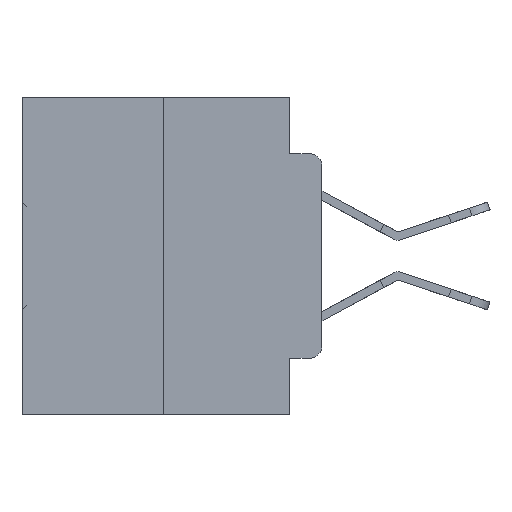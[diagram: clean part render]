
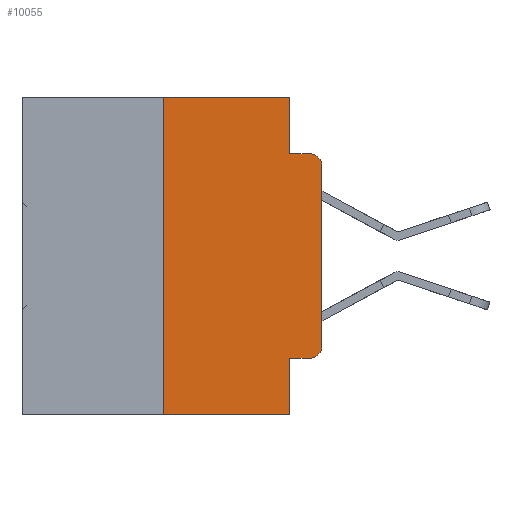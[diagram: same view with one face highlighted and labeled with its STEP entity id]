
A CAD part, left-side view. The second image highlights one B-rep face of the part: STEP entity #10055.
In plain terms, the highlighted planar face has unit normal (-1, 0, 0).
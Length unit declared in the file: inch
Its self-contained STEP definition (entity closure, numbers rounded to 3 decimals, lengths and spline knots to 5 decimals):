
#95 = VECTOR ( 'NONE', #13742, 39.37008 ) ;
#285 = LINE ( 'NONE', #8115, #6824 ) ;
#997 = DIRECTION ( 'NONE',  ( 0., 0., -1. ) ) ;
#1004 = AXIS2_PLACEMENT_3D ( 'NONE', #31628, #31731, #15728 ) ;
#1594 = LINE ( 'NONE', #14963, #7240 ) ;
#1630 = CARTESIAN_POINT ( 'NONE',  ( 0., 0.051, 0. ) ) ;
#1645 = VECTOR ( 'NONE', #19854, 39.37008 ) ;
#3509 = DIRECTION ( 'NONE',  ( 0., -1., 0. ) ) ;
#4352 = EDGE_CURVE ( 'NONE', #29738, #25983, #16354, .T. ) ;
#5220 = DIRECTION ( 'NONE',  ( 0., 0., -1. ) ) ;
#5519 = DIRECTION ( 'NONE',  ( -1., 0., 0. ) ) ;
#6055 = CARTESIAN_POINT ( 'NONE',  ( 0., 0., 0. ) ) ;
#6824 = VECTOR ( 'NONE', #5220, 39.37008 ) ;
#6904 = EDGE_CURVE ( 'NONE', #14923, #12381, #17433, .T. ) ;
#7240 = VECTOR ( 'NONE', #17704, 39.37008 ) ;
#7461 = EDGE_CURVE ( 'NONE', #29738, #15882, #28268, .T. ) ;
#7504 = LINE ( 'NONE', #32410, #95 ) ;
#7684 = CARTESIAN_POINT ( 'NONE',  ( 0., 0.25, -0.5 ) ) ;
#8115 = CARTESIAN_POINT ( 'NONE',  ( 0., 0.051, 0. ) ) ;
#8301 = VECTOR ( 'NONE', #27364, 39.37008 ) ;
#8988 = FACE_OUTER_BOUND ( 'NONE', #20516, .T. ) ;
#9211 = AXIS2_PLACEMENT_3D ( 'NONE', #21919, #5519, #24635 ) ;
#9593 = VERTEX_POINT ( 'NONE', #24716 ) ;
#9876 = CARTESIAN_POINT ( 'NONE',  ( 0., 0.25, 0. ) ) ;
#10055 = ADVANCED_FACE ( 'NONE', ( #8988 ), #29065, .F. ) ;
#10080 = VERTEX_POINT ( 'NONE', #26545 ) ;
#10403 = ORIENTED_EDGE ( 'NONE', *, *, #17963, .F. ) ;
#11167 = CARTESIAN_POINT ( 'NONE',  ( 0., 0.051, -0.4115 ) ) ;
#12381 = VERTEX_POINT ( 'NONE', #28707 ) ;
#13608 = EDGE_CURVE ( 'NONE', #19005, #15882, #16886, .T. ) ;
#13742 = DIRECTION ( 'NONE',  ( 0., -1., 0. ) ) ;
#13770 = LINE ( 'NONE', #6055, #27266 ) ;
#13833 = VERTEX_POINT ( 'NONE', #15984 ) ;
#13845 = ORIENTED_EDGE ( 'NONE', *, *, #28698, .F. ) ;
#14912 = DIRECTION ( 'NONE',  ( 0., 0., -1. ) ) ;
#14923 = VERTEX_POINT ( 'NONE', #23714 ) ;
#14963 = CARTESIAN_POINT ( 'NONE',  ( 0., 0.473, 0. ) ) ;
#15728 = DIRECTION ( 'NONE',  ( 0., 0., -1. ) ) ;
#15882 = VERTEX_POINT ( 'NONE', #30179 ) ;
#15984 = CARTESIAN_POINT ( 'NONE',  ( 0., 0., -0.3915 ) ) ;
#16354 = LINE ( 'NONE', #22711, #1645 ) ;
#16886 = LINE ( 'NONE', #28288, #30284 ) ;
#16978 = ORIENTED_EDGE ( 'NONE', *, *, #33406, .T. ) ;
#17433 = CIRCLE ( 'NONE', #32794, 0.02 ) ;
#17547 = DIRECTION ( 'NONE',  ( -1., 0., 0. ) ) ;
#17704 = DIRECTION ( 'NONE',  ( 0., -1., 0. ) ) ;
#17963 = EDGE_CURVE ( 'NONE', #9593, #12381, #7504, .T. ) ;
#18576 = ORIENTED_EDGE ( 'NONE', *, *, #4352, .F. ) ;
#19005 = VERTEX_POINT ( 'NONE', #34560 ) ;
#19854 = DIRECTION ( 'NONE',  ( 0., 0., 1. ) ) ;
#19982 = CARTESIAN_POINT ( 'NONE',  ( 0., 0.473, -0.5 ) ) ;
#20516 = EDGE_LOOP ( 'NONE', ( #33984, #29403, #10403, #13845, #22763, #18576, #27401, #34906, #27432, #16978 ) ) ;
#20984 = CIRCLE ( 'NONE', #9211, 0.02 ) ;
#21197 = VECTOR ( 'NONE', #3509, 39.37008 ) ;
#21919 = CARTESIAN_POINT ( 'NONE',  ( 0., 0.02, -0.3915 ) ) ;
#22711 = CARTESIAN_POINT ( 'NONE',  ( 0., 0.25, 0. ) ) ;
#22763 = ORIENTED_EDGE ( 'NONE', *, *, #28954, .F. ) ;
#23660 = LINE ( 'NONE', #11167, #8301 ) ;
#23714 = CARTESIAN_POINT ( 'NONE',  ( 0., 0., -0.1085 ) ) ;
#24635 = DIRECTION ( 'NONE',  ( 0., 0., -1. ) ) ;
#24716 = CARTESIAN_POINT ( 'NONE',  ( 0., 0.051, -0.0885 ) ) ;
#25983 = VERTEX_POINT ( 'NONE', #9876 ) ;
#26304 = EDGE_CURVE ( 'NONE', #19005, #10080, #23660, .T. ) ;
#26545 = CARTESIAN_POINT ( 'NONE',  ( 0., 0.02, -0.4115 ) ) ;
#27266 = VECTOR ( 'NONE', #27775, 39.37008 ) ;
#27364 = DIRECTION ( 'NONE',  ( 0., -1., 0. ) ) ;
#27401 = ORIENTED_EDGE ( 'NONE', *, *, #7461, .T. ) ;
#27432 = ORIENTED_EDGE ( 'NONE', *, *, #26304, .T. ) ;
#27775 = DIRECTION ( 'NONE',  ( 0., 0., 1. ) ) ;
#27786 = VERTEX_POINT ( 'NONE', #1630 ) ;
#28268 = LINE ( 'NONE', #19982, #21197 ) ;
#28288 = CARTESIAN_POINT ( 'NONE',  ( 0., 0.051, 0. ) ) ;
#28698 = EDGE_CURVE ( 'NONE', #27786, #9593, #285, .T. ) ;
#28707 = CARTESIAN_POINT ( 'NONE',  ( 0., 0.02, -0.0885 ) ) ;
#28954 = EDGE_CURVE ( 'NONE', #25983, #27786, #1594, .T. ) ;
#29065 = PLANE ( 'NONE',  #1004 ) ;
#29403 = ORIENTED_EDGE ( 'NONE', *, *, #6904, .T. ) ;
#29738 = VERTEX_POINT ( 'NONE', #7684 ) ;
#30179 = CARTESIAN_POINT ( 'NONE',  ( 0., 0.051, -0.5 ) ) ;
#30284 = VECTOR ( 'NONE', #14912, 39.37008 ) ;
#31628 = CARTESIAN_POINT ( 'NONE',  ( 0., 0.473, 0. ) ) ;
#31731 = DIRECTION ( 'NONE',  ( 1., 0., 0. ) ) ;
#32410 = CARTESIAN_POINT ( 'NONE',  ( 0., 0.051, -0.0885 ) ) ;
#32794 = AXIS2_PLACEMENT_3D ( 'NONE', #33545, #17547, #997 ) ;
#32936 = EDGE_CURVE ( 'NONE', #13833, #14923, #13770, .T. ) ;
#33406 = EDGE_CURVE ( 'NONE', #10080, #13833, #20984, .T. ) ;
#33545 = CARTESIAN_POINT ( 'NONE',  ( 0., 0.02, -0.1085 ) ) ;
#33984 = ORIENTED_EDGE ( 'NONE', *, *, #32936, .T. ) ;
#34560 = CARTESIAN_POINT ( 'NONE',  ( 0., 0.051, -0.4115 ) ) ;
#34906 = ORIENTED_EDGE ( 'NONE', *, *, #13608, .F. ) ;
